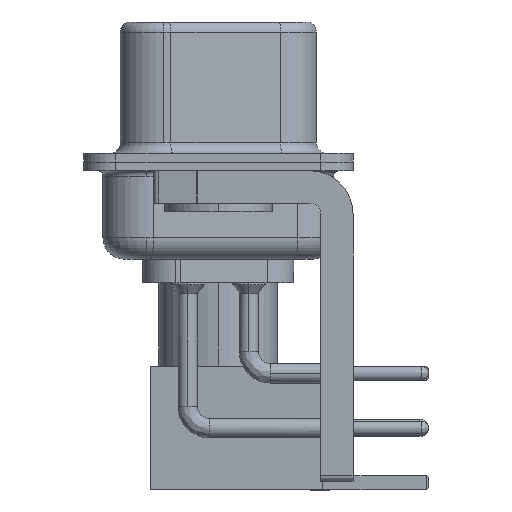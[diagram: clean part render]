
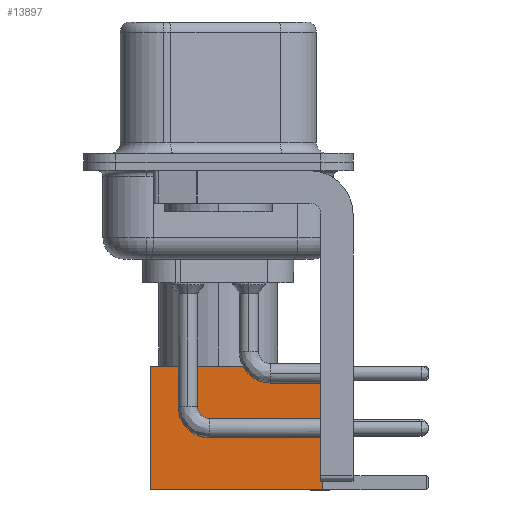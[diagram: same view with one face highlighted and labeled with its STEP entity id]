
A CAD part, left-side view. The second image highlights one B-rep face of the part: STEP entity #13897.
In plain terms, the highlighted face is planar.
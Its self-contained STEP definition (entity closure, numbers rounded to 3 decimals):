
#212 = LINE ( 'NONE', #7648, #8615 ) ;
#1163 = EDGE_CURVE ( 'NONE', #9026, #11430, #20024, .T. ) ;
#1258 = VERTEX_POINT ( 'NONE', #20257 ) ;
#2641 = LINE ( 'NONE', #21280, #5496 ) ;
#2861 = CARTESIAN_POINT ( 'NONE',  ( -2.875, 2.875, 0. ) ) ;
#3950 = CARTESIAN_POINT ( 'NONE',  ( -2.875, 2.875, 8. ) ) ;
#4080 = EDGE_CURVE ( 'NONE', #11830, #1258, #4732, .T. ) ;
#4732 = LINE ( 'NONE', #6195, #15554 ) ;
#5091 = FACE_OUTER_BOUND ( 'NONE', #10891, .T. ) ;
#5153 = VECTOR ( 'NONE', #21367, 1000. ) ;
#5496 = VECTOR ( 'NONE', #5942, 1000. ) ;
#5852 = EDGE_CURVE ( 'NONE', #11830, #9026, #212, .T. ) ;
#5942 = DIRECTION ( 'NONE',  ( -1., 0., 0. ) ) ;
#6195 = CARTESIAN_POINT ( 'NONE',  ( 2.875, 2.875, 0. ) ) ;
#6655 = ORIENTED_EDGE ( 'NONE', *, *, #5852, .F. ) ;
#7648 = CARTESIAN_POINT ( 'NONE',  ( 0., 2.875, 8. ) ) ;
#8398 = PLANE ( 'NONE',  #13269 ) ;
#8615 = VECTOR ( 'NONE', #13363, 1000. ) ;
#9026 = VERTEX_POINT ( 'NONE', #3950 ) ;
#10216 = DIRECTION ( 'NONE',  ( 0., 0., -1. ) ) ;
#10891 = EDGE_LOOP ( 'NONE', ( #21158, #12307, #21726, #6655 ) ) ;
#11430 = VERTEX_POINT ( 'NONE', #18701 ) ;
#11830 = VERTEX_POINT ( 'NONE', #16847 ) ;
#12307 = ORIENTED_EDGE ( 'NONE', *, *, #14262, .T. ) ;
#13269 = AXIS2_PLACEMENT_3D ( 'NONE', #16298, #19610, #15825 ) ;
#13363 = DIRECTION ( 'NONE',  ( -1., 0., 0. ) ) ;
#13897 = ADVANCED_FACE ( 'NONE', ( #5091 ), #8398, .T. ) ;
#14262 = EDGE_CURVE ( 'NONE', #1258, #11430, #2641, .T. ) ;
#15554 = VECTOR ( 'NONE', #10216, 1000. ) ;
#15825 = DIRECTION ( 'NONE',  ( 0., 0., 1. ) ) ;
#16298 = CARTESIAN_POINT ( 'NONE',  ( 2.875, 2.875, 0. ) ) ;
#16847 = CARTESIAN_POINT ( 'NONE',  ( 2.875, 2.875, 8. ) ) ;
#18701 = CARTESIAN_POINT ( 'NONE',  ( -2.875, 2.875, 0. ) ) ;
#19610 = DIRECTION ( 'NONE',  ( 0., 1., 0. ) ) ;
#20024 = LINE ( 'NONE', #2861, #5153 ) ;
#20257 = CARTESIAN_POINT ( 'NONE',  ( 2.875, 2.875, 0. ) ) ;
#21158 = ORIENTED_EDGE ( 'NONE', *, *, #4080, .T. ) ;
#21280 = CARTESIAN_POINT ( 'NONE',  ( 0., 2.875, 0. ) ) ;
#21367 = DIRECTION ( 'NONE',  ( 0., 0., -1. ) ) ;
#21726 = ORIENTED_EDGE ( 'NONE', *, *, #1163, .F. ) ;
